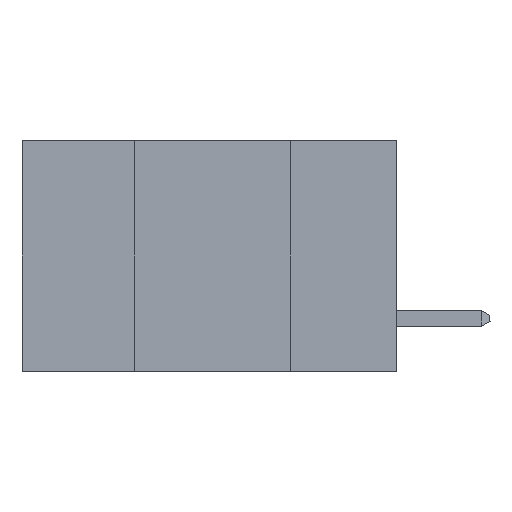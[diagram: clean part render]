
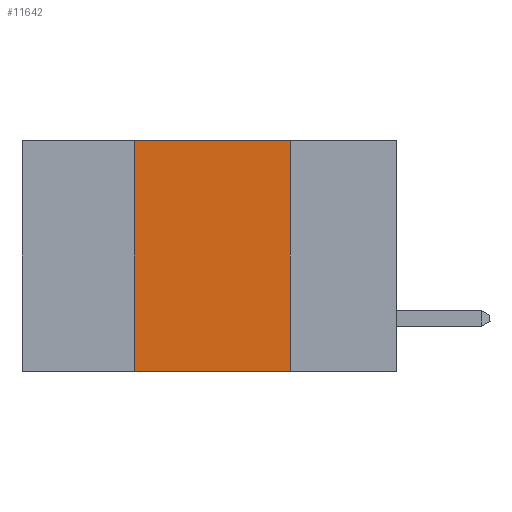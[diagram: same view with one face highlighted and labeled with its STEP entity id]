
A CAD part, left-side view. The second image highlights one B-rep face of the part: STEP entity #11642.
In plain terms, the highlighted planar face has unit normal (-1, 0, 0).
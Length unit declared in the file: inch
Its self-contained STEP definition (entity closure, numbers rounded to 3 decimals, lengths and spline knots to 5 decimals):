
#515 = VERTEX_POINT ( 'NONE', #4524 ) ;
#873 = DIRECTION ( 'NONE',  ( 0., 0., -1. ) ) ;
#1433 = LINE ( 'NONE', #12960, #15891 ) ;
#1882 = CARTESIAN_POINT ( 'NONE',  ( 0., 0.6, 0. ) ) ;
#2471 = VERTEX_POINT ( 'NONE', #12256 ) ;
#3189 = VECTOR ( 'NONE', #14750, 39.37008 ) ;
#3482 = CARTESIAN_POINT ( 'NONE',  ( 0., 0.17, 0. ) ) ;
#4122 = EDGE_CURVE ( 'NONE', #515, #2471, #1433, .T. ) ;
#4524 = CARTESIAN_POINT ( 'NONE',  ( 0., 0.42, -0.37 ) ) ;
#4729 = CARTESIAN_POINT ( 'NONE',  ( 0., 0.6, 0. ) ) ;
#4886 = LINE ( 'NONE', #3482, #7481 ) ;
#4912 = EDGE_LOOP ( 'NONE', ( #6958, #7374, #9307, #12267 ) ) ;
#6721 = EDGE_CURVE ( 'NONE', #2471, #9536, #9935, .T. ) ;
#6958 = ORIENTED_EDGE ( 'NONE', *, *, #12622, .F. ) ;
#7374 = ORIENTED_EDGE ( 'NONE', *, *, #6721, .F. ) ;
#7378 = DIRECTION ( 'NONE',  ( 1., 0., 0. ) ) ;
#7481 = VECTOR ( 'NONE', #873, 39.37008 ) ;
#7522 = LINE ( 'NONE', #9331, #13849 ) ;
#8091 = CARTESIAN_POINT ( 'NONE',  ( 0., 0.17, 0. ) ) ;
#8366 = AXIS2_PLACEMENT_3D ( 'NONE', #4729, #7378, #16295 ) ;
#8492 = CARTESIAN_POINT ( 'NONE',  ( 0., 0.17, -0.37 ) ) ;
#8588 = VERTEX_POINT ( 'NONE', #8492 ) ;
#9307 = ORIENTED_EDGE ( 'NONE', *, *, #4122, .F. ) ;
#9331 = CARTESIAN_POINT ( 'NONE',  ( 0., 0.6, -0.37 ) ) ;
#9536 = VERTEX_POINT ( 'NONE', #8091 ) ;
#9540 = EDGE_CURVE ( 'NONE', #515, #8588, #7522, .T. ) ;
#9622 = DIRECTION ( 'NONE',  ( 0., 0., 1. ) ) ;
#9935 = LINE ( 'NONE', #1882, #3189 ) ;
#10582 = DIRECTION ( 'NONE',  ( 0., -1., 0. ) ) ;
#11642 = ADVANCED_FACE ( 'NONE', ( #12818 ), #14992, .F. ) ;
#12256 = CARTESIAN_POINT ( 'NONE',  ( 0., 0.42, 0. ) ) ;
#12267 = ORIENTED_EDGE ( 'NONE', *, *, #9540, .T. ) ;
#12622 = EDGE_CURVE ( 'NONE', #9536, #8588, #4886, .T. ) ;
#12818 = FACE_OUTER_BOUND ( 'NONE', #4912, .T. ) ;
#12960 = CARTESIAN_POINT ( 'NONE',  ( 0., 0.42, 0. ) ) ;
#13849 = VECTOR ( 'NONE', #10582, 39.37008 ) ;
#14750 = DIRECTION ( 'NONE',  ( 0., -1., 0. ) ) ;
#14992 = PLANE ( 'NONE',  #8366 ) ;
#15891 = VECTOR ( 'NONE', #9622, 39.37008 ) ;
#16295 = DIRECTION ( 'NONE',  ( 0., 0., -1. ) ) ;
